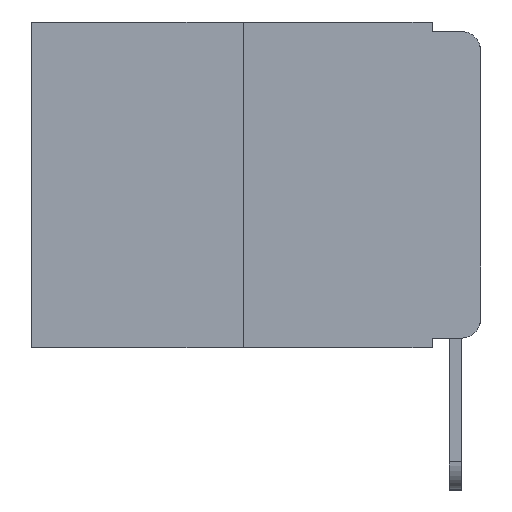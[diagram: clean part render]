
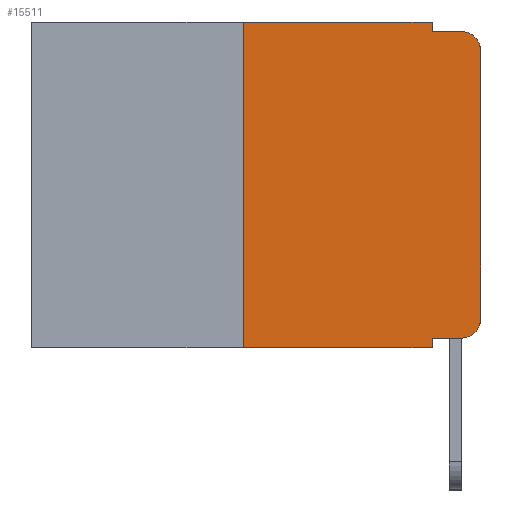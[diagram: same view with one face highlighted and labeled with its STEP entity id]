
A CAD part, left-side view. The second image highlights one B-rep face of the part: STEP entity #15511.
In plain terms, the highlighted planar face has unit normal (-1, 0, 0).
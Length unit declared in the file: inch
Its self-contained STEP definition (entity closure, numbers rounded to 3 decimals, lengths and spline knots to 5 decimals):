
#83 = CARTESIAN_POINT ( 'NONE',  ( 0., 0.473, 0. ) ) ;
#480 = AXIS2_PLACEMENT_3D ( 'NONE', #83, #3677, #15219 ) ;
#887 = CARTESIAN_POINT ( 'NONE',  ( 0., 0.02, -0.313 ) ) ;
#1171 = LINE ( 'NONE', #6435, #18696 ) ;
#1724 = EDGE_LOOP ( 'NONE', ( #5918, #3546, #21252, #15707, #3328, #11954, #12213, #10419, #9112, #2538 ) ) ;
#1735 = EDGE_CURVE ( 'NONE', #10504, #15327, #9083, .T. ) ;
#1893 = CARTESIAN_POINT ( 'NONE',  ( 0., 0.25, 0. ) ) ;
#2175 = CARTESIAN_POINT ( 'NONE',  ( 0., 0.051, -0.01 ) ) ;
#2538 = ORIENTED_EDGE ( 'NONE', *, *, #6282, .T. ) ;
#2617 = DIRECTION ( 'NONE',  ( 0., 0., -1. ) ) ;
#3051 = CARTESIAN_POINT ( 'NONE',  ( 0., 0.25, 0. ) ) ;
#3215 = VECTOR ( 'NONE', #19119, 39.37008 ) ;
#3328 = ORIENTED_EDGE ( 'NONE', *, *, #6436, .F. ) ;
#3503 = VERTEX_POINT ( 'NONE', #18527 ) ;
#3546 = ORIENTED_EDGE ( 'NONE', *, *, #21072, .T. ) ;
#3600 = DIRECTION ( 'NONE',  ( 0., 0., 1. ) ) ;
#3677 = DIRECTION ( 'NONE',  ( 1., 0., 0. ) ) ;
#3776 = CARTESIAN_POINT ( 'NONE',  ( 0., 0.051, -0.01 ) ) ;
#3832 = VERTEX_POINT ( 'NONE', #19366 ) ;
#4439 = EDGE_CURVE ( 'NONE', #8881, #7381, #20509, .T. ) ;
#5918 = ORIENTED_EDGE ( 'NONE', *, *, #20085, .T. ) ;
#6105 = DIRECTION ( 'NONE',  ( -1., 0., 0. ) ) ;
#6282 = EDGE_CURVE ( 'NONE', #15327, #7117, #20171, .T. ) ;
#6435 = CARTESIAN_POINT ( 'NONE',  ( 0., 0.051, 0. ) ) ;
#6436 = EDGE_CURVE ( 'NONE', #21239, #3503, #20389, .T. ) ;
#7043 = CARTESIAN_POINT ( 'NONE',  ( 0., 0., -0.03 ) ) ;
#7117 = VERTEX_POINT ( 'NONE', #20540 ) ;
#7381 = VERTEX_POINT ( 'NONE', #9923 ) ;
#7549 = CARTESIAN_POINT ( 'NONE',  ( 0., 0., 0. ) ) ;
#7752 = VECTOR ( 'NONE', #19753, 39.37008 ) ;
#8258 = LINE ( 'NONE', #18168, #7752 ) ;
#8540 = AXIS2_PLACEMENT_3D ( 'NONE', #887, #12588, #2617 ) ;
#8556 = VECTOR ( 'NONE', #18736, 39.37008 ) ;
#8881 = VERTEX_POINT ( 'NONE', #3776 ) ;
#9003 = LINE ( 'NONE', #7549, #13384 ) ;
#9083 = LINE ( 'NONE', #19286, #8556 ) ;
#9112 = ORIENTED_EDGE ( 'NONE', *, *, #1735, .T. ) ;
#9923 = CARTESIAN_POINT ( 'NONE',  ( 0., 0.02, -0.01 ) ) ;
#10419 = ORIENTED_EDGE ( 'NONE', *, *, #19719, .F. ) ;
#10504 = VERTEX_POINT ( 'NONE', #14285 ) ;
#11120 = EDGE_CURVE ( 'NONE', #3503, #8881, #1171, .T. ) ;
#11679 = CARTESIAN_POINT ( 'NONE',  ( 0., 0.473, 0. ) ) ;
#11954 = ORIENTED_EDGE ( 'NONE', *, *, #15468, .F. ) ;
#11964 = VECTOR ( 'NONE', #21133, 39.37008 ) ;
#12213 = ORIENTED_EDGE ( 'NONE', *, *, #16841, .T. ) ;
#12464 = CARTESIAN_POINT ( 'NONE',  ( 0., 0.25, -0.343 ) ) ;
#12523 = DIRECTION ( 'NONE',  ( 0., 0., 1. ) ) ;
#12588 = DIRECTION ( 'NONE',  ( -1., 0., 0. ) ) ;
#13245 = CARTESIAN_POINT ( 'NONE',  ( 0., 0.02, -0.333 ) ) ;
#13384 = VECTOR ( 'NONE', #12523, 39.37008 ) ;
#13600 = PLANE ( 'NONE',  #480 ) ;
#14285 = CARTESIAN_POINT ( 'NONE',  ( 0., 0.051, -0.333 ) ) ;
#14313 = VECTOR ( 'NONE', #19669, 39.37008 ) ;
#15219 = DIRECTION ( 'NONE',  ( 0., 0., -1. ) ) ;
#15327 = VERTEX_POINT ( 'NONE', #13245 ) ;
#15468 = EDGE_CURVE ( 'NONE', #19425, #21239, #20661, .T. ) ;
#15511 = ADVANCED_FACE ( 'NONE', ( #15541 ), #13600, .F. ) ;
#15541 = FACE_OUTER_BOUND ( 'NONE', #1724, .T. ) ;
#15707 = ORIENTED_EDGE ( 'NONE', *, *, #11120, .F. ) ;
#15898 = CARTESIAN_POINT ( 'NONE',  ( 0., 0.02, -0.03 ) ) ;
#16034 = VECTOR ( 'NONE', #3600, 39.37008 ) ;
#16695 = AXIS2_PLACEMENT_3D ( 'NONE', #15898, #6105, #17498 ) ;
#16841 = EDGE_CURVE ( 'NONE', #19425, #3832, #8258, .T. ) ;
#17498 = DIRECTION ( 'NONE',  ( 0., 0., -1. ) ) ;
#17594 = CIRCLE ( 'NONE', #16695, 0.02 ) ;
#17816 = DIRECTION ( 'NONE',  ( 0., 0., -1. ) ) ;
#18168 = CARTESIAN_POINT ( 'NONE',  ( 0., 0.473, -0.343 ) ) ;
#18527 = CARTESIAN_POINT ( 'NONE',  ( 0., 0.051, 0. ) ) ;
#18696 = VECTOR ( 'NONE', #17816, 39.37008 ) ;
#18736 = DIRECTION ( 'NONE',  ( 0., -1., 0. ) ) ;
#19073 = LINE ( 'NONE', #21209, #14313 ) ;
#19119 = DIRECTION ( 'NONE',  ( 0., -1., 0. ) ) ;
#19286 = CARTESIAN_POINT ( 'NONE',  ( 0., 0.051, -0.333 ) ) ;
#19366 = CARTESIAN_POINT ( 'NONE',  ( 0., 0.051, -0.343 ) ) ;
#19425 = VERTEX_POINT ( 'NONE', #12464 ) ;
#19669 = DIRECTION ( 'NONE',  ( 0., 0., -1. ) ) ;
#19719 = EDGE_CURVE ( 'NONE', #10504, #3832, #19073, .T. ) ;
#19753 = DIRECTION ( 'NONE',  ( 0., -1., 0. ) ) ;
#20085 = EDGE_CURVE ( 'NONE', #7117, #20603, #9003, .T. ) ;
#20171 = CIRCLE ( 'NONE', #8540, 0.02 ) ;
#20389 = LINE ( 'NONE', #11679, #11964 ) ;
#20509 = LINE ( 'NONE', #2175, #3215 ) ;
#20540 = CARTESIAN_POINT ( 'NONE',  ( 0., 0., -0.313 ) ) ;
#20603 = VERTEX_POINT ( 'NONE', #7043 ) ;
#20661 = LINE ( 'NONE', #1893, #16034 ) ;
#21072 = EDGE_CURVE ( 'NONE', #20603, #7381, #17594, .T. ) ;
#21133 = DIRECTION ( 'NONE',  ( 0., -1., 0. ) ) ;
#21209 = CARTESIAN_POINT ( 'NONE',  ( 0., 0.051, 0. ) ) ;
#21239 = VERTEX_POINT ( 'NONE', #3051 ) ;
#21252 = ORIENTED_EDGE ( 'NONE', *, *, #4439, .F. ) ;
